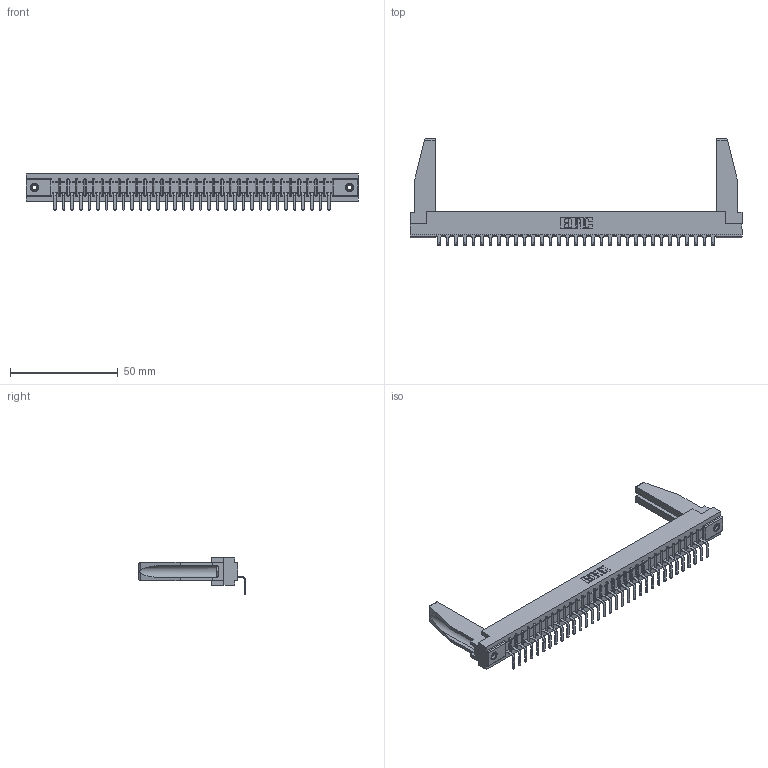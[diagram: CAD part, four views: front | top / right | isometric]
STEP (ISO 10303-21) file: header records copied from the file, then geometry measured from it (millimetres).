
FILE_DESCRIPTION (( 'STEP AP203' ), '1' );
FILE_NAME ('307-033-559-178.STEP', '2019-09-05T16:43:28', ( '' ), ( '' ), 'SwSTEP 2.0', 'SolidWorks 2016', '' );
FILE_SCHEMA (( 'CONFIG_CONTROL_DESIGN' ));
Length unit declared in the file: inch
Products named in the file (5): 307-220-078; 307-290-001_558 559 - 1 (Single); 307-033-559-178; 307 Part_.156 Dia Mounting Holes; 345-250-001_345-250-001-102
Assembly tree (38 placements, depth 2):
  307-033-559-178
    307 Part_.156 Dia Mounting Holes
    307-290-001_558 559 - 1 (Single)  x33
    307-220-078  x2
    345-250-001_345-250-001-102  x2
Bounding box: 153.77 x 49.16 x 16.8 mm (x, y, z)
Volume: 19945.7 mm3; surface area: 20852.4 mm2
Topology: 38 solids, 38 shells, 2262 faces, 6395 edges, 4118 vertices
Faces by surface type: plane 1441, cylinder 737, sphere 68, cone 12, torus 4
Entity records: 31943 total; most frequent: CARTESIAN_POINT 5378, ORIENTED_EDGE 5320, DIRECTION 5192, EDGE_CURVE 2660, VECTOR 2040, LINE 2040, VERTEX_POINT 1720, AXIS2_PLACEMENT_3D 1576
